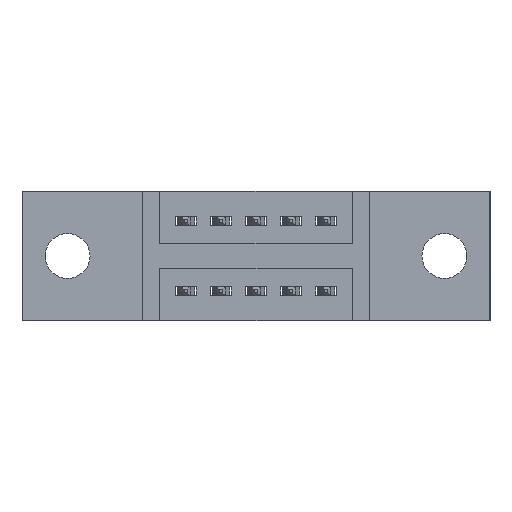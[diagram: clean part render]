
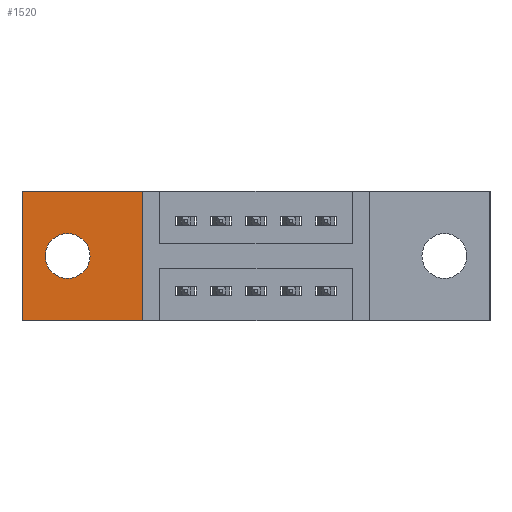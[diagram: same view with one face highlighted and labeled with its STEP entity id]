
A CAD part, front view. The second image highlights one B-rep face of the part: STEP entity #1520.
In plain terms, the highlighted planar face has unit normal (0, -1, 0).
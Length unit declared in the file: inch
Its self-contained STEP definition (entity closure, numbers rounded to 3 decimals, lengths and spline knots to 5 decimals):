
#40 = DIRECTION ( 'NONE',  ( 0., 0., -1. ) ) ;
#92 = EDGE_CURVE ( 'NONE', #7567, #5094, #6507, .T. ) ;
#174 = CARTESIAN_POINT ( 'NONE',  ( 0., 0.11, 0. ) ) ;
#566 = CARTESIAN_POINT ( 'NONE',  ( 0., 0.11, 0. ) ) ;
#593 = CIRCLE ( 'NONE', #3456, 0.064 ) ;
#627 = VECTOR ( 'NONE', #6763, 39.37008 ) ;
#654 = EDGE_CURVE ( 'NONE', #4333, #2250, #8156, .T. ) ;
#813 = DIRECTION ( 'NONE',  ( 0., 0., -1. ) ) ;
#1069 = EDGE_CURVE ( 'NONE', #4001, #4333, #3404, .T. ) ;
#1175 = CARTESIAN_POINT ( 'NONE',  ( 0.13, 0.11, -0.185 ) ) ;
#1183 = FACE_OUTER_BOUND ( 'NONE', #4278, .T. ) ;
#1244 = VECTOR ( 'NONE', #5021, 39.37008 ) ;
#1520 = ADVANCED_FACE ( 'NONE', ( #6904, #1183 ), #2169, .T. ) ;
#1554 = AXIS2_PLACEMENT_3D ( 'NONE', #2273, #7859, #813 ) ;
#1959 = EDGE_CURVE ( 'NONE', #5094, #7567, #593, .T. ) ;
#2169 = PLANE ( 'NONE',  #5046 ) ;
#2200 = DIRECTION ( 'NONE',  ( 0., -1., 0. ) ) ;
#2250 = VERTEX_POINT ( 'NONE', #5206 ) ;
#2273 = CARTESIAN_POINT ( 'NONE',  ( 0.13, 0.11, -0.185 ) ) ;
#3137 = DIRECTION ( 'NONE',  ( 0., -1., 0. ) ) ;
#3247 = CARTESIAN_POINT ( 'NONE',  ( 0.3425, 0.11, 0. ) ) ;
#3297 = VECTOR ( 'NONE', #8337, 39.37008 ) ;
#3404 = LINE ( 'NONE', #174, #8570 ) ;
#3456 = AXIS2_PLACEMENT_3D ( 'NONE', #1175, #3137, #8761 ) ;
#3466 = ORIENTED_EDGE ( 'NONE', *, *, #7568, .T. ) ;
#3541 = ORIENTED_EDGE ( 'NONE', *, *, #654, .T. ) ;
#3552 = CARTESIAN_POINT ( 'NONE',  ( 0., 0.11, -0.37 ) ) ;
#3634 = CARTESIAN_POINT ( 'NONE',  ( 0.3425, 0.11, 0. ) ) ;
#3945 = CARTESIAN_POINT ( 'NONE',  ( 0.3425, 0.11, -0.37 ) ) ;
#4001 = VERTEX_POINT ( 'NONE', #3247 ) ;
#4260 = ORIENTED_EDGE ( 'NONE', *, *, #92, .F. ) ;
#4263 = CARTESIAN_POINT ( 'NONE',  ( 0.13, 0.11, -0.249 ) ) ;
#4278 = EDGE_LOOP ( 'NONE', ( #3541, #7729, #3466, #7195 ) ) ;
#4333 = VERTEX_POINT ( 'NONE', #566 ) ;
#4590 = EDGE_LOOP ( 'NONE', ( #4260, #5368 ) ) ;
#4692 = CARTESIAN_POINT ( 'NONE',  ( 0., 0.11, -0.37 ) ) ;
#5021 = DIRECTION ( 'NONE',  ( 0., 0., 1. ) ) ;
#5046 = AXIS2_PLACEMENT_3D ( 'NONE', #3552, #2200, #40 ) ;
#5094 = VERTEX_POINT ( 'NONE', #4263 ) ;
#5206 = CARTESIAN_POINT ( 'NONE',  ( 0., 0.11, -0.37 ) ) ;
#5368 = ORIENTED_EDGE ( 'NONE', *, *, #1959, .F. ) ;
#5472 = CARTESIAN_POINT ( 'NONE',  ( 0., 0.11, 0. ) ) ;
#6449 = CARTESIAN_POINT ( 'NONE',  ( 0.13, 0.11, -0.121 ) ) ;
#6486 = DIRECTION ( 'NONE',  ( -1., 0., 0. ) ) ;
#6507 = CIRCLE ( 'NONE', #1554, 0.064 ) ;
#6545 = EDGE_CURVE ( 'NONE', #2250, #7094, #6588, .T. ) ;
#6588 = LINE ( 'NONE', #4692, #627 ) ;
#6763 = DIRECTION ( 'NONE',  ( 1., 0., 0. ) ) ;
#6904 = FACE_BOUND ( 'NONE', #4590, .T. ) ;
#7094 = VERTEX_POINT ( 'NONE', #3945 ) ;
#7195 = ORIENTED_EDGE ( 'NONE', *, *, #1069, .T. ) ;
#7532 = LINE ( 'NONE', #3634, #1244 ) ;
#7567 = VERTEX_POINT ( 'NONE', #6449 ) ;
#7568 = EDGE_CURVE ( 'NONE', #7094, #4001, #7532, .T. ) ;
#7729 = ORIENTED_EDGE ( 'NONE', *, *, #6545, .T. ) ;
#7859 = DIRECTION ( 'NONE',  ( 0., -1., 0. ) ) ;
#8156 = LINE ( 'NONE', #5472, #3297 ) ;
#8337 = DIRECTION ( 'NONE',  ( 0., 0., -1. ) ) ;
#8570 = VECTOR ( 'NONE', #6486, 39.37008 ) ;
#8761 = DIRECTION ( 'NONE',  ( 0., 0., -1. ) ) ;
